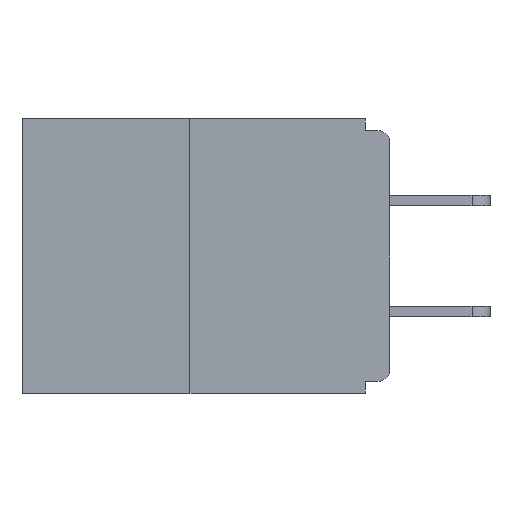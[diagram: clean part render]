
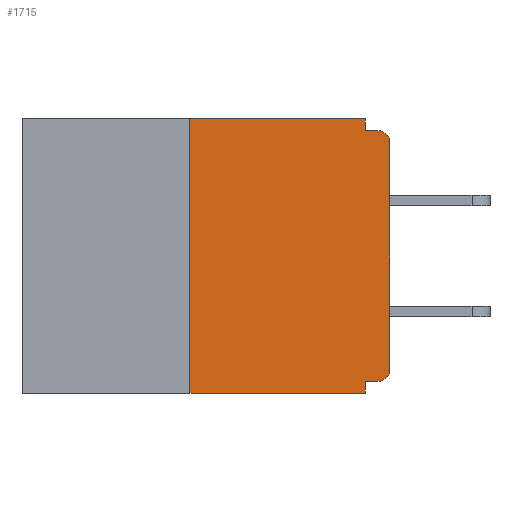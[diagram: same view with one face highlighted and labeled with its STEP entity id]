
A CAD part, left-side view. The second image highlights one B-rep face of the part: STEP entity #1715.
In plain terms, the highlighted planar face has unit normal (-1, 0, 0).
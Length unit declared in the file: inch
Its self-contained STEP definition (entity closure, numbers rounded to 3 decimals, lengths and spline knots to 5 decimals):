
#101 = CARTESIAN_POINT ( 'NONE',  ( 0., 0.031, -0.343 ) ) ;
#225 = AXIS2_PLACEMENT_3D ( 'NONE', #3826, #13565, #6245 ) ;
#338 = EDGE_CURVE ( 'NONE', #2846, #13723, #12498, .T. ) ;
#659 = AXIS2_PLACEMENT_3D ( 'NONE', #8962, #12753, #6660 ) ;
#960 = VERTEX_POINT ( 'NONE', #11953 ) ;
#1581 = CARTESIAN_POINT ( 'NONE',  ( 0., 0.031, 0. ) ) ;
#1655 = EDGE_CURVE ( 'NONE', #9361, #1750, #3724, .T. ) ;
#1715 = ADVANCED_FACE ( 'NONE', ( #9407 ), #7410, .F. ) ;
#1750 = VERTEX_POINT ( 'NONE', #6354 ) ;
#1807 = ORIENTED_EDGE ( 'NONE', *, *, #3287, .F. ) ;
#2208 = LINE ( 'NONE', #15257, #13437 ) ;
#2257 = ORIENTED_EDGE ( 'NONE', *, *, #14903, .T. ) ;
#2325 = ORIENTED_EDGE ( 'NONE', *, *, #14414, .F. ) ;
#2700 = DIRECTION ( 'NONE',  ( 0., 0., -1. ) ) ;
#2735 = VECTOR ( 'NONE', #4299, 39.37008 ) ;
#2846 = VERTEX_POINT ( 'NONE', #11807 ) ;
#3085 = CARTESIAN_POINT ( 'NONE',  ( 0., 0., -0.328 ) ) ;
#3210 = VERTEX_POINT ( 'NONE', #14887 ) ;
#3287 = EDGE_CURVE ( 'NONE', #13723, #4163, #5768, .T. ) ;
#3463 = CARTESIAN_POINT ( 'NONE',  ( 0., 0.015, -0.313 ) ) ;
#3538 = CARTESIAN_POINT ( 'NONE',  ( 0., 0.25, -0.343 ) ) ;
#3724 = LINE ( 'NONE', #8487, #11130 ) ;
#3823 = ORIENTED_EDGE ( 'NONE', *, *, #6543, .F. ) ;
#3826 = CARTESIAN_POINT ( 'NONE',  ( 0., 0.46, 0. ) ) ;
#3945 = CARTESIAN_POINT ( 'NONE',  ( 0., 0.46, -0.343 ) ) ;
#4163 = VERTEX_POINT ( 'NONE', #14130 ) ;
#4235 = ORIENTED_EDGE ( 'NONE', *, *, #1655, .T. ) ;
#4299 = DIRECTION ( 'NONE',  ( 0., 1., 0. ) ) ;
#4821 = VECTOR ( 'NONE', #2700, 39.37008 ) ;
#4857 = CARTESIAN_POINT ( 'NONE',  ( 0., 0.015, -0.328 ) ) ;
#5008 = DIRECTION ( 'NONE',  ( 0., 0., -1. ) ) ;
#5035 = ORIENTED_EDGE ( 'NONE', *, *, #10456, .T. ) ;
#5118 = CIRCLE ( 'NONE', #8653, 0.015 ) ;
#5768 = LINE ( 'NONE', #1581, #4821 ) ;
#5973 = CARTESIAN_POINT ( 'NONE',  ( 0., 0., -0.313 ) ) ;
#6245 = DIRECTION ( 'NONE',  ( 0., 0., -1. ) ) ;
#6354 = CARTESIAN_POINT ( 'NONE',  ( 0., 0., -0.03 ) ) ;
#6412 = EDGE_CURVE ( 'NONE', #4163, #960, #2208, .T. ) ;
#6543 = EDGE_CURVE ( 'NONE', #8536, #2846, #9409, .T. ) ;
#6584 = CARTESIAN_POINT ( 'NONE',  ( 0., 0.46, 0. ) ) ;
#6660 = DIRECTION ( 'NONE',  ( 0., 0., -1. ) ) ;
#7410 = PLANE ( 'NONE',  #225 ) ;
#7492 = ORIENTED_EDGE ( 'NONE', *, *, #338, .F. ) ;
#7862 = VERTEX_POINT ( 'NONE', #11933 ) ;
#8487 = CARTESIAN_POINT ( 'NONE',  ( 0., 0., 0. ) ) ;
#8536 = VERTEX_POINT ( 'NONE', #3538 ) ;
#8653 = AXIS2_PLACEMENT_3D ( 'NONE', #3463, #14377, #15658 ) ;
#8962 = CARTESIAN_POINT ( 'NONE',  ( 0., 0.015, -0.03 ) ) ;
#9361 = VERTEX_POINT ( 'NONE', #5973 ) ;
#9407 = FACE_OUTER_BOUND ( 'NONE', #10240, .T. ) ;
#9409 = LINE ( 'NONE', #12023, #10734 ) ;
#10240 = EDGE_LOOP ( 'NONE', ( #7492, #3823, #2257, #2325, #14207, #5035, #4235, #13521, #13364, #1807 ) ) ;
#10456 = EDGE_CURVE ( 'NONE', #13821, #9361, #5118, .T. ) ;
#10665 = LINE ( 'NONE', #101, #15653 ) ;
#10683 = DIRECTION ( 'NONE',  ( 0., 0., 1. ) ) ;
#10734 = VECTOR ( 'NONE', #10683, 39.37008 ) ;
#10957 = EDGE_CURVE ( 'NONE', #1750, #960, #14449, .T. ) ;
#11130 = VECTOR ( 'NONE', #13411, 39.37008 ) ;
#11807 = CARTESIAN_POINT ( 'NONE',  ( 0., 0.25, 0. ) ) ;
#11933 = CARTESIAN_POINT ( 'NONE',  ( 0., 0.031, -0.328 ) ) ;
#11953 = CARTESIAN_POINT ( 'NONE',  ( 0., 0.015, -0.015 ) ) ;
#12023 = CARTESIAN_POINT ( 'NONE',  ( 0., 0.25, 0. ) ) ;
#12369 = VECTOR ( 'NONE', #12839, 39.37008 ) ;
#12498 = LINE ( 'NONE', #6584, #13095 ) ;
#12753 = DIRECTION ( 'NONE',  ( -1., 0., 0. ) ) ;
#12796 = DIRECTION ( 'NONE',  ( 0., -1., 0. ) ) ;
#12839 = DIRECTION ( 'NONE',  ( 0., -1., 0. ) ) ;
#13095 = VECTOR ( 'NONE', #15094, 39.37008 ) ;
#13325 = LINE ( 'NONE', #3945, #12369 ) ;
#13364 = ORIENTED_EDGE ( 'NONE', *, *, #6412, .F. ) ;
#13406 = EDGE_CURVE ( 'NONE', #13821, #7862, #15505, .T. ) ;
#13411 = DIRECTION ( 'NONE',  ( 0., 0., 1. ) ) ;
#13437 = VECTOR ( 'NONE', #12796, 39.37008 ) ;
#13521 = ORIENTED_EDGE ( 'NONE', *, *, #10957, .T. ) ;
#13565 = DIRECTION ( 'NONE',  ( 1., 0., 0. ) ) ;
#13723 = VERTEX_POINT ( 'NONE', #15780 ) ;
#13821 = VERTEX_POINT ( 'NONE', #4857 ) ;
#14130 = CARTESIAN_POINT ( 'NONE',  ( 0., 0.031, -0.015 ) ) ;
#14207 = ORIENTED_EDGE ( 'NONE', *, *, #13406, .F. ) ;
#14377 = DIRECTION ( 'NONE',  ( -1., 0., 0. ) ) ;
#14414 = EDGE_CURVE ( 'NONE', #7862, #3210, #10665, .T. ) ;
#14449 = CIRCLE ( 'NONE', #659, 0.015 ) ;
#14887 = CARTESIAN_POINT ( 'NONE',  ( 0., 0.031, -0.343 ) ) ;
#14903 = EDGE_CURVE ( 'NONE', #8536, #3210, #13325, .T. ) ;
#15094 = DIRECTION ( 'NONE',  ( 0., -1., 0. ) ) ;
#15257 = CARTESIAN_POINT ( 'NONE',  ( 0., 0., -0.015 ) ) ;
#15505 = LINE ( 'NONE', #3085, #2735 ) ;
#15653 = VECTOR ( 'NONE', #5008, 39.37008 ) ;
#15658 = DIRECTION ( 'NONE',  ( 0., 0., -1. ) ) ;
#15780 = CARTESIAN_POINT ( 'NONE',  ( 0., 0.031, 0. ) ) ;
